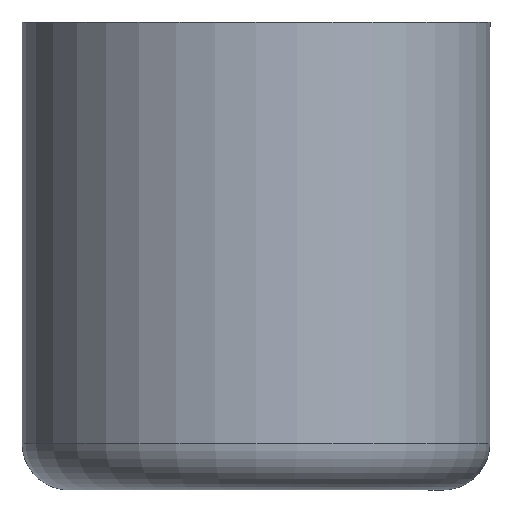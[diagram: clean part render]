
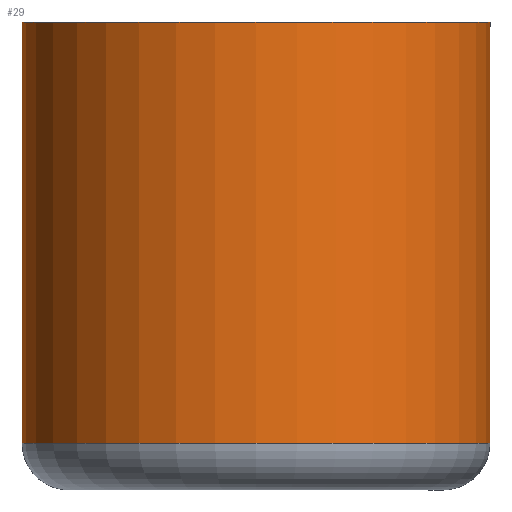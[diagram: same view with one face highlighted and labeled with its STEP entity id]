
A CAD part, front view. The second image highlights one B-rep face of the part: STEP entity #29.
In plain terms, the highlighted cylindrical face has radius 5 mm (diameter 10 mm), a partial arc.
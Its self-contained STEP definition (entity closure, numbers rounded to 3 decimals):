
#13 = CIRCLE ( 'NONE', #137, 5. ) ;
#19 = LINE ( 'NONE', #108, #116 ) ;
#29 = ADVANCED_FACE ( 'NONE', ( #102 ), #245, .T. ) ;
#33 = ORIENTED_EDGE ( 'NONE', *, *, #246, .F. ) ;
#37 = VERTEX_POINT ( 'NONE', #203 ) ;
#39 = CIRCLE ( 'NONE', #127, 5. ) ;
#44 = VECTOR ( 'NONE', #183, 1000. ) ;
#53 = ORIENTED_EDGE ( 'NONE', *, *, #267, .T. ) ;
#55 = EDGE_LOOP ( 'NONE', ( #33, #206, #79, #53 ) ) ;
#79 = ORIENTED_EDGE ( 'NONE', *, *, #269, .T. ) ;
#81 = VERTEX_POINT ( 'NONE', #150 ) ;
#102 = FACE_OUTER_BOUND ( 'NONE', #55, .T. ) ;
#105 = DIRECTION ( 'NONE',  ( 0., 0., -1. ) ) ;
#106 = CARTESIAN_POINT ( 'NONE',  ( 0., 0., 10. ) ) ;
#107 = DIRECTION ( 'NONE',  ( -1., 0., 0. ) ) ;
#108 = CARTESIAN_POINT ( 'NONE',  ( 5., 0., 0. ) ) ;
#109 = DIRECTION ( 'NONE',  ( 0., 0., 1. ) ) ;
#116 = VECTOR ( 'NONE', #258, 1000. ) ;
#121 = VERTEX_POINT ( 'NONE', #197 ) ;
#124 = CARTESIAN_POINT ( 'NONE',  ( 0., 0., 1. ) ) ;
#127 = AXIS2_PLACEMENT_3D ( 'NONE', #106, #105, #107 ) ;
#131 = CARTESIAN_POINT ( 'NONE',  ( -5., 0., 10. ) ) ;
#133 = CARTESIAN_POINT ( 'NONE',  ( 0., 0., 0. ) ) ;
#137 = AXIS2_PLACEMENT_3D ( 'NONE', #124, #141, #148 ) ;
#141 = DIRECTION ( 'NONE',  ( 0., 0., 1. ) ) ;
#148 = DIRECTION ( 'NONE',  ( -1., 0., 0. ) ) ;
#150 = CARTESIAN_POINT ( 'NONE',  ( -5., 0., 1. ) ) ;
#160 = DIRECTION ( 'NONE',  ( 1., 0., 0. ) ) ;
#183 = DIRECTION ( 'NONE',  ( 0., 0., 1. ) ) ;
#190 = AXIS2_PLACEMENT_3D ( 'NONE', #133, #109, #160 ) ;
#195 = CARTESIAN_POINT ( 'NONE',  ( -5., 0., 0. ) ) ;
#197 = CARTESIAN_POINT ( 'NONE',  ( 5., 0., 1. ) ) ;
#203 = CARTESIAN_POINT ( 'NONE',  ( 5., 0., 10. ) ) ;
#206 = ORIENTED_EDGE ( 'NONE', *, *, #264, .T. ) ;
#245 = CYLINDRICAL_SURFACE ( 'NONE', #190, 5. ) ;
#246 = EDGE_CURVE ( 'NONE', #81, #263, #249, .T. ) ;
#249 = LINE ( 'NONE', #195, #44 ) ;
#258 = DIRECTION ( 'NONE',  ( 0., 0., 1. ) ) ;
#263 = VERTEX_POINT ( 'NONE', #131 ) ;
#264 = EDGE_CURVE ( 'NONE', #81, #121, #13, .T. ) ;
#267 = EDGE_CURVE ( 'NONE', #37, #263, #39, .T. ) ;
#269 = EDGE_CURVE ( 'NONE', #121, #37, #19, .T. ) ;
